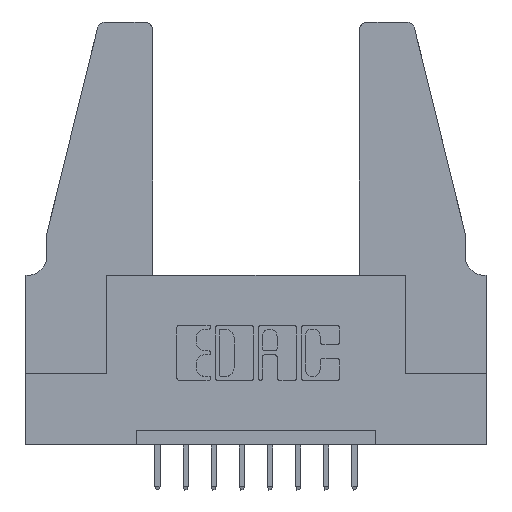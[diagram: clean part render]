
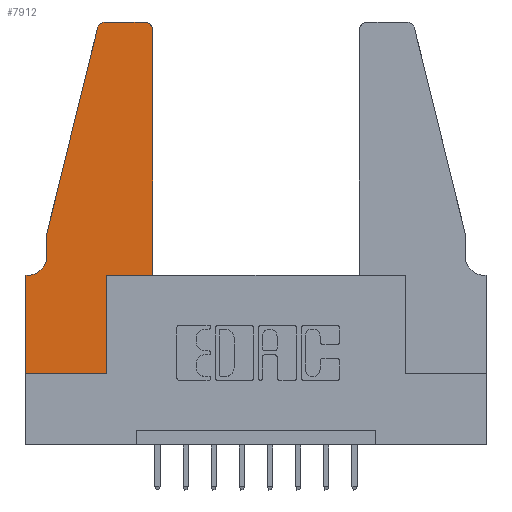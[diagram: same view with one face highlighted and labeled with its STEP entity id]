
A CAD part, top view. The second image highlights one B-rep face of the part: STEP entity #7912.
In plain terms, the highlighted planar face has unit normal (0, 0, 1).
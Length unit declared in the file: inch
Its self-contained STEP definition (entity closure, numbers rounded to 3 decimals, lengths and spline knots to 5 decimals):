
#350 = DIRECTION ( 'NONE',  ( 1., 0., 0. ) ) ;
#530 = VECTOR ( 'NONE', #10018, 39.37008 ) ;
#578 = CARTESIAN_POINT ( 'NONE',  ( 0.4205, 1.22, 0.37 ) ) ;
#648 = VECTOR ( 'NONE', #3707, 39.37008 ) ;
#837 = DIRECTION ( 'NONE',  ( 0., -1., 0. ) ) ;
#981 = DIRECTION ( 'NONE',  ( 1., 0., 0. ) ) ;
#1056 = VECTOR ( 'NONE', #5093, 39.37008 ) ;
#1421 = CARTESIAN_POINT ( 'NONE',  ( 0., 0.35, 0.37 ) ) ;
#1515 = ORIENTED_EDGE ( 'NONE', *, *, #3068, .T. ) ;
#1634 = VERTEX_POINT ( 'NONE', #10716 ) ;
#1752 = FACE_OUTER_BOUND ( 'NONE', #3150, .T. ) ;
#1774 = VERTEX_POINT ( 'NONE', #11031 ) ;
#1895 = DIRECTION ( 'NONE',  ( 0., 0., -1. ) ) ;
#1919 = CARTESIAN_POINT ( 'NONE',  ( 0.0755, 0.42, 0.37 ) ) ;
#2122 = ORIENTED_EDGE ( 'NONE', *, *, #6897, .T. ) ;
#2274 = EDGE_CURVE ( 'NONE', #9555, #10137, #9668, .T. ) ;
#2296 = DIRECTION ( 'NONE',  ( 0., 0., 1. ) ) ;
#2348 = CARTESIAN_POINT ( 'NONE',  ( 0., 0., 0.37 ) ) ;
#2673 = LINE ( 'NONE', #10304, #7156 ) ;
#2767 = CARTESIAN_POINT ( 'NONE',  ( 0.4205, 1.25, 0.37 ) ) ;
#2787 = VECTOR ( 'NONE', #10257, 39.37008 ) ;
#2926 = AXIS2_PLACEMENT_3D ( 'NONE', #12022, #3933, #981 ) ;
#3068 = EDGE_CURVE ( 'NONE', #9208, #1774, #3733, .T. ) ;
#3150 = EDGE_LOOP ( 'NONE', ( #2122, #8935, #3532, #6195, #3161, #5857, #1515, #8759, #6012, #9686, #4231, #5973 ) ) ;
#3161 = ORIENTED_EDGE ( 'NONE', *, *, #11434, .T. ) ;
#3326 = EDGE_CURVE ( 'NONE', #11479, #1634, #2673, .T. ) ;
#3452 = VECTOR ( 'NONE', #11837, 39.37008 ) ;
#3532 = ORIENTED_EDGE ( 'NONE', *, *, #3326, .T. ) ;
#3707 = DIRECTION ( 'NONE',  ( 0., 1., 0. ) ) ;
#3733 = LINE ( 'NONE', #6016, #4193 ) ;
#3789 = VERTEX_POINT ( 'NONE', #4958 ) ;
#3802 = CARTESIAN_POINT ( 'NONE',  ( 0.0055, 0.42, 0.37 ) ) ;
#3933 = DIRECTION ( 'NONE',  ( 0., 0., 1. ) ) ;
#4091 = CARTESIAN_POINT ( 'NONE',  ( 0.4505, 0.35, 0.37 ) ) ;
#4099 = CIRCLE ( 'NONE', #2926, 0.03 ) ;
#4193 = VECTOR ( 'NONE', #12023, 39.37008 ) ;
#4213 = LINE ( 'NONE', #5689, #12770 ) ;
#4231 = ORIENTED_EDGE ( 'NONE', *, *, #4728, .T. ) ;
#4595 = DIRECTION ( 'NONE',  ( 0., 0., 1. ) ) ;
#4728 = EDGE_CURVE ( 'NONE', #10137, #5865, #5036, .T. ) ;
#4852 = CARTESIAN_POINT ( 'NONE',  ( 0.4505, 0.35, 0.37 ) ) ;
#4958 = CARTESIAN_POINT ( 'NONE',  ( 0.2865, 0., 0.37 ) ) ;
#5036 = LINE ( 'NONE', #4091, #1056 ) ;
#5093 = DIRECTION ( 'NONE',  ( 0., 1., 0. ) ) ;
#5238 = CARTESIAN_POINT ( 'NONE',  ( 0.0755, 0.35, 0.37 ) ) ;
#5689 = CARTESIAN_POINT ( 'NONE',  ( 0.0755, 0.5, 0.37 ) ) ;
#5857 = ORIENTED_EDGE ( 'NONE', *, *, #9180, .T. ) ;
#5865 = VERTEX_POINT ( 'NONE', #11755 ) ;
#5973 = ORIENTED_EDGE ( 'NONE', *, *, #11961, .T. ) ;
#6012 = ORIENTED_EDGE ( 'NONE', *, *, #11900, .T. ) ;
#6016 = CARTESIAN_POINT ( 'NONE',  ( 0., 0., 0.37 ) ) ;
#6195 = ORIENTED_EDGE ( 'NONE', *, *, #7007, .T. ) ;
#6652 = CARTESIAN_POINT ( 'NONE',  ( 0.2865, 0.35, 0.37 ) ) ;
#6897 = EDGE_CURVE ( 'NONE', #12567, #8001, #8106, .T. ) ;
#7007 = EDGE_CURVE ( 'NONE', #1634, #12719, #4213, .T. ) ;
#7156 = VECTOR ( 'NONE', #10170, 39.37008 ) ;
#7246 = AXIS2_PLACEMENT_3D ( 'NONE', #578, #4595, #11576 ) ;
#7311 = DIRECTION ( 'NONE',  ( 1., 0., 0. ) ) ;
#7912 = ADVANCED_FACE ( 'NONE', ( #1752 ), #9174, .T. ) ;
#8001 = VERTEX_POINT ( 'NONE', #9126 ) ;
#8106 = LINE ( 'NONE', #9935, #530 ) ;
#8146 = AXIS2_PLACEMENT_3D ( 'NONE', #3802, #1895, #9671 ) ;
#8337 = LINE ( 'NONE', #2348, #11625 ) ;
#8743 = CARTESIAN_POINT ( 'NONE',  ( 0.25487, 1.22718, 0.37 ) ) ;
#8759 = ORIENTED_EDGE ( 'NONE', *, *, #9590, .T. ) ;
#8935 = ORIENTED_EDGE ( 'NONE', *, *, #10334, .T. ) ;
#9126 = CARTESIAN_POINT ( 'NONE',  ( 0.284, 1.25, 0.37 ) ) ;
#9174 = PLANE ( 'NONE',  #10297 ) ;
#9180 = EDGE_CURVE ( 'NONE', #12434, #9208, #11175, .T. ) ;
#9208 = VERTEX_POINT ( 'NONE', #1421 ) ;
#9356 = CARTESIAN_POINT ( 'NONE',  ( 0.0055, 0.35, 0.37 ) ) ;
#9446 = CARTESIAN_POINT ( 'NONE',  ( 0.2865, 0.35, 0.37 ) ) ;
#9555 = VERTEX_POINT ( 'NONE', #9446 ) ;
#9590 = EDGE_CURVE ( 'NONE', #1774, #3789, #8337, .T. ) ;
#9626 = LINE ( 'NONE', #6652, #648 ) ;
#9668 = LINE ( 'NONE', #4852, #3452 ) ;
#9671 = DIRECTION ( 'NONE',  ( -1., 0., 0. ) ) ;
#9686 = ORIENTED_EDGE ( 'NONE', *, *, #2274, .T. ) ;
#9935 = CARTESIAN_POINT ( 'NONE',  ( 0.2605, 1.25, 0.37 ) ) ;
#10018 = DIRECTION ( 'NONE',  ( -1., 0., 0. ) ) ;
#10137 = VERTEX_POINT ( 'NONE', #10748 ) ;
#10170 = DIRECTION ( 'NONE',  ( -0.239, -0.971, 0. ) ) ;
#10257 = DIRECTION ( 'NONE',  ( -1., 0., 0. ) ) ;
#10297 = AXIS2_PLACEMENT_3D ( 'NONE', #12098, #2296, #350 ) ;
#10304 = CARTESIAN_POINT ( 'NONE',  ( 0.0755, 0.5, 0.37 ) ) ;
#10334 = EDGE_CURVE ( 'NONE', #8001, #11479, #4099, .T. ) ;
#10435 = CIRCLE ( 'NONE', #8146, 0.07 ) ;
#10570 = CIRCLE ( 'NONE', #7246, 0.03 ) ;
#10716 = CARTESIAN_POINT ( 'NONE',  ( 0.0755, 0.5, 0.37 ) ) ;
#10748 = CARTESIAN_POINT ( 'NONE',  ( 0.4505, 0.35, 0.37 ) ) ;
#11031 = CARTESIAN_POINT ( 'NONE',  ( 0., 0., 0.37 ) ) ;
#11175 = LINE ( 'NONE', #5238, #2787 ) ;
#11434 = EDGE_CURVE ( 'NONE', #12719, #12434, #10435, .T. ) ;
#11479 = VERTEX_POINT ( 'NONE', #8743 ) ;
#11576 = DIRECTION ( 'NONE',  ( 1., 0., 0. ) ) ;
#11625 = VECTOR ( 'NONE', #7311, 39.37008 ) ;
#11755 = CARTESIAN_POINT ( 'NONE',  ( 0.4505, 1.22, 0.37 ) ) ;
#11837 = DIRECTION ( 'NONE',  ( 1., 0., 0. ) ) ;
#11900 = EDGE_CURVE ( 'NONE', #3789, #9555, #9626, .T. ) ;
#11961 = EDGE_CURVE ( 'NONE', #5865, #12567, #10570, .T. ) ;
#12022 = CARTESIAN_POINT ( 'NONE',  ( 0.284, 1.22, 0.37 ) ) ;
#12023 = DIRECTION ( 'NONE',  ( 0., -1., 0. ) ) ;
#12098 = CARTESIAN_POINT ( 'NONE',  ( 0., 0.35, 0.37 ) ) ;
#12434 = VERTEX_POINT ( 'NONE', #9356 ) ;
#12567 = VERTEX_POINT ( 'NONE', #2767 ) ;
#12719 = VERTEX_POINT ( 'NONE', #1919 ) ;
#12770 = VECTOR ( 'NONE', #837, 39.37008 ) ;
